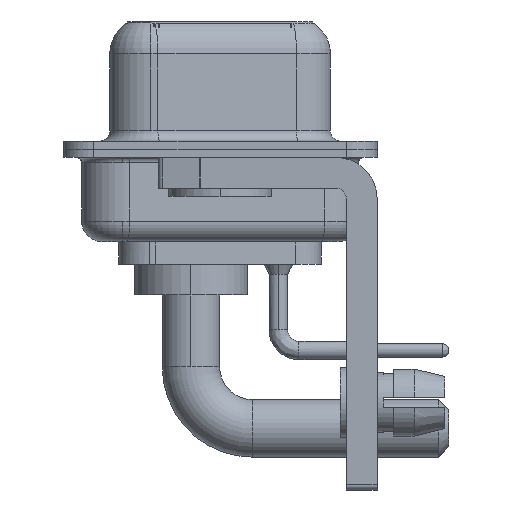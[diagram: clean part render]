
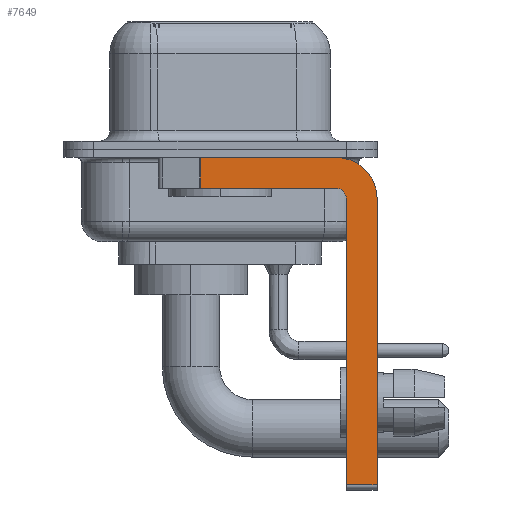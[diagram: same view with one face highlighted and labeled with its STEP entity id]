
A CAD part, left-side view. The second image highlights one B-rep face of the part: STEP entity #7649.
In plain terms, the highlighted planar face has unit normal (-1, 0, 0).
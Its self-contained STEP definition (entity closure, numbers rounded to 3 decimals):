
#159 = CARTESIAN_POINT ( 'NONE',  ( -2.9, -6.15, -16.6 ) ) ;
#250 = ORIENTED_EDGE ( 'NONE', *, *, #13110, .F. ) ;
#270 = LINE ( 'NONE', #159, #8173 ) ;
#393 = VERTEX_POINT ( 'NONE', #1373 ) ;
#402 = CARTESIAN_POINT ( 'NONE',  ( -2.9, 0.978, -1.9 ) ) ;
#698 = AXIS2_PLACEMENT_3D ( 'NONE', #7507, #10978, #14813 ) ;
#1373 = CARTESIAN_POINT ( 'NONE',  ( -2.9, -5.65, -0.4 ) ) ;
#1427 = CARTESIAN_POINT ( 'NONE',  ( -2.9, -6.15, -2.4 ) ) ;
#1454 = VERTEX_POINT ( 'NONE', #19366 ) ;
#2553 = ORIENTED_EDGE ( 'NONE', *, *, #7849, .F. ) ;
#2573 = CIRCLE ( 'NONE', #20158, 2. ) ;
#2801 = CARTESIAN_POINT ( 'NONE',  ( -2.9, -5.65, -16.35 ) ) ;
#3208 = DIRECTION ( 'NONE',  ( 0., 1., 0. ) ) ;
#3233 = VERTEX_POINT ( 'NONE', #5734 ) ;
#3692 = EDGE_CURVE ( 'NONE', #7599, #3233, #10229, .T. ) ;
#4586 = CARTESIAN_POINT ( 'NONE',  ( -2.9, 0.978, -1.9 ) ) ;
#4872 = EDGE_LOOP ( 'NONE', ( #250, #21755, #9977, #11882, #23362, #12595, #2553, #5364 ) ) ;
#4985 = CARTESIAN_POINT ( 'NONE',  ( -2.9, -5.65, -1.9 ) ) ;
#5181 = VERTEX_POINT ( 'NONE', #11462 ) ;
#5364 = ORIENTED_EDGE ( 'NONE', *, *, #7972, .F. ) ;
#5734 = CARTESIAN_POINT ( 'NONE',  ( -2.9, -5.65, -1.9 ) ) ;
#6400 = VECTOR ( 'NONE', #3208, 1000. ) ;
#6658 = DIRECTION ( 'NONE',  ( 1., 0., 0. ) ) ;
#6706 = VERTEX_POINT ( 'NONE', #17850 ) ;
#6865 = CARTESIAN_POINT ( 'NONE',  ( -2.9, -6.15, -16.35 ) ) ;
#7047 = PLANE ( 'NONE',  #7517 ) ;
#7507 = CARTESIAN_POINT ( 'NONE',  ( -2.9, -5.65, -2.4 ) ) ;
#7517 = AXIS2_PLACEMENT_3D ( 'NONE', #21994, #20319, #12683 ) ;
#7599 = VERTEX_POINT ( 'NONE', #1427 ) ;
#7649 = ADVANCED_FACE ( 'NONE', ( #8948 ), #7047, .F. ) ;
#7849 = EDGE_CURVE ( 'NONE', #6706, #5181, #15168, .T. ) ;
#7972 = EDGE_CURVE ( 'NONE', #393, #6706, #2573, .T. ) ;
#8017 = EDGE_CURVE ( 'NONE', #3233, #22405, #14217, .T. ) ;
#8173 = VECTOR ( 'NONE', #14730, 1000. ) ;
#8445 = CARTESIAN_POINT ( 'NONE',  ( -2.9, -5.65, -2.4 ) ) ;
#8666 = VERTEX_POINT ( 'NONE', #6865 ) ;
#8948 = FACE_OUTER_BOUND ( 'NONE', #4872, .T. ) ;
#9345 = LINE ( 'NONE', #402, #15688 ) ;
#9977 = ORIENTED_EDGE ( 'NONE', *, *, #8017, .F. ) ;
#10229 = CIRCLE ( 'NONE', #698, 0.5 ) ;
#10447 = DIRECTION ( 'NONE',  ( 0., -1., 0. ) ) ;
#10978 = DIRECTION ( 'NONE',  ( -1., 0., 0. ) ) ;
#11033 = LINE ( 'NONE', #12953, #22905 ) ;
#11462 = CARTESIAN_POINT ( 'NONE',  ( -2.9, -7.65, -16.35 ) ) ;
#11882 = ORIENTED_EDGE ( 'NONE', *, *, #3692, .F. ) ;
#12595 = ORIENTED_EDGE ( 'NONE', *, *, #15778, .T. ) ;
#12683 = DIRECTION ( 'NONE',  ( 0., 0., -1. ) ) ;
#12953 = CARTESIAN_POINT ( 'NONE',  ( -2.9, 3., -0.4 ) ) ;
#13110 = EDGE_CURVE ( 'NONE', #1454, #393, #11033, .T. ) ;
#13735 = DIRECTION ( 'NONE',  ( 0., 0., -1. ) ) ;
#14057 = EDGE_CURVE ( 'NONE', #1454, #22405, #9345, .T. ) ;
#14217 = LINE ( 'NONE', #4985, #6400 ) ;
#14730 = DIRECTION ( 'NONE',  ( 0., 0., 1. ) ) ;
#14813 = DIRECTION ( 'NONE',  ( 0., 0., 1. ) ) ;
#14988 = VECTOR ( 'NONE', #10447, 1000. ) ;
#15168 = LINE ( 'NONE', #17057, #19729 ) ;
#15688 = VECTOR ( 'NONE', #16647, 1000. ) ;
#15778 = EDGE_CURVE ( 'NONE', #8666, #5181, #19529, .T. ) ;
#16647 = DIRECTION ( 'NONE',  ( 0., 0., -1. ) ) ;
#16649 = DIRECTION ( 'NONE',  ( 0., -1., 0. ) ) ;
#17057 = CARTESIAN_POINT ( 'NONE',  ( -2.9, -7.65, -2.4 ) ) ;
#17850 = CARTESIAN_POINT ( 'NONE',  ( -2.9, -7.65, -2.4 ) ) ;
#18561 = EDGE_CURVE ( 'NONE', #8666, #7599, #270, .T. ) ;
#18747 = DIRECTION ( 'NONE',  ( 0., 0., -1. ) ) ;
#19366 = CARTESIAN_POINT ( 'NONE',  ( -2.9, 0.978, -0.4 ) ) ;
#19529 = LINE ( 'NONE', #2801, #14988 ) ;
#19729 = VECTOR ( 'NONE', #18747, 1000. ) ;
#20158 = AXIS2_PLACEMENT_3D ( 'NONE', #8445, #6658, #13735 ) ;
#20319 = DIRECTION ( 'NONE',  ( 1., 0., 0. ) ) ;
#21755 = ORIENTED_EDGE ( 'NONE', *, *, #14057, .T. ) ;
#21994 = CARTESIAN_POINT ( 'NONE',  ( -2.9, -5.65, -2.4 ) ) ;
#22405 = VERTEX_POINT ( 'NONE', #4586 ) ;
#22905 = VECTOR ( 'NONE', #16649, 1000. ) ;
#23362 = ORIENTED_EDGE ( 'NONE', *, *, #18561, .F. ) ;
